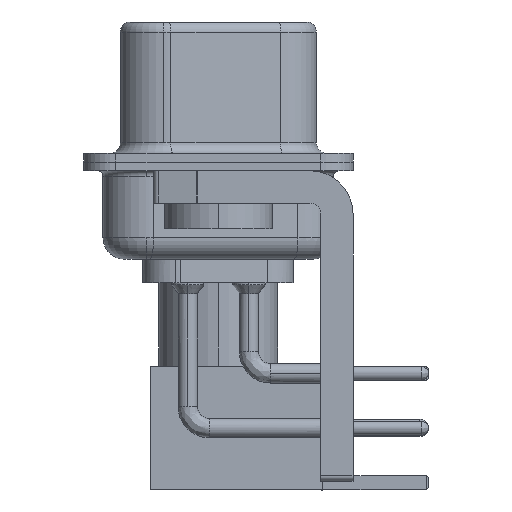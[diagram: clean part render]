
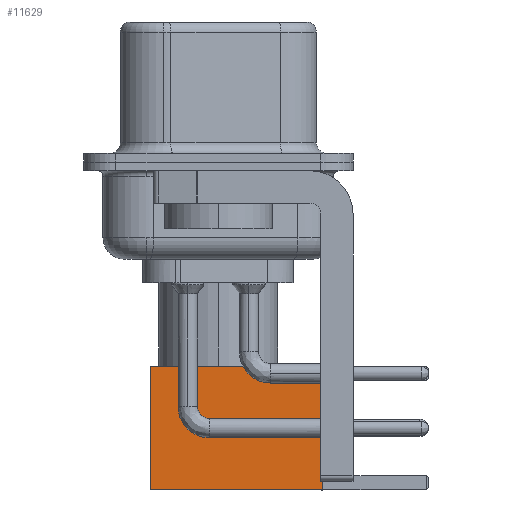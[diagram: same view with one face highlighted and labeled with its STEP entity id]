
A CAD part, left-side view. The second image highlights one B-rep face of the part: STEP entity #11629.
In plain terms, the highlighted face is planar.
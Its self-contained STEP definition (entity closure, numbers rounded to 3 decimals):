
#339 = EDGE_CURVE ( 'NONE', #1229, #10793, #1042, .T. ) ;
#400 = CARTESIAN_POINT ( 'NONE',  ( 2.875, 2.875, 0. ) ) ;
#430 = VECTOR ( 'NONE', #20013, 1000. ) ;
#1042 = LINE ( 'NONE', #17690, #430 ) ;
#1229 = VERTEX_POINT ( 'NONE', #17886 ) ;
#2007 = VECTOR ( 'NONE', #15887, 1000. ) ;
#2085 = CARTESIAN_POINT ( 'NONE',  ( 2.875, 2.875, 8. ) ) ;
#2715 = DIRECTION ( 'NONE',  ( 0., 0., 1. ) ) ;
#3270 = VERTEX_POINT ( 'NONE', #13412 ) ;
#3455 = CARTESIAN_POINT ( 'NONE',  ( 0., 2.875, 8. ) ) ;
#5475 = AXIS2_PLACEMENT_3D ( 'NONE', #400, #17496, #2715 ) ;
#10328 = LINE ( 'NONE', #3455, #12085 ) ;
#10793 = VERTEX_POINT ( 'NONE', #30194 ) ;
#11629 = ADVANCED_FACE ( 'NONE', ( #21705 ), #14875, .T. ) ;
#12078 = EDGE_CURVE ( 'NONE', #19626, #1229, #30085, .T. ) ;
#12085 = VECTOR ( 'NONE', #13126, 1000. ) ;
#12333 = LINE ( 'NONE', #14365, #27071 ) ;
#12868 = ORIENTED_EDGE ( 'NONE', *, *, #12078, .T. ) ;
#13126 = DIRECTION ( 'NONE',  ( -1., 0., 0. ) ) ;
#13412 = CARTESIAN_POINT ( 'NONE',  ( -2.875, 2.875, 8. ) ) ;
#14365 = CARTESIAN_POINT ( 'NONE',  ( -2.875, 2.875, 0. ) ) ;
#14718 = EDGE_CURVE ( 'NONE', #19626, #3270, #10328, .T. ) ;
#14875 = PLANE ( 'NONE',  #5475 ) ;
#15887 = DIRECTION ( 'NONE',  ( 0., 0., -1. ) ) ;
#16580 = ORIENTED_EDGE ( 'NONE', *, *, #339, .T. ) ;
#16824 = EDGE_CURVE ( 'NONE', #3270, #10793, #12333, .T. ) ;
#17496 = DIRECTION ( 'NONE',  ( 0., 1., 0. ) ) ;
#17690 = CARTESIAN_POINT ( 'NONE',  ( 0., 2.875, 0. ) ) ;
#17886 = CARTESIAN_POINT ( 'NONE',  ( 2.875, 2.875, 0. ) ) ;
#19626 = VERTEX_POINT ( 'NONE', #2085 ) ;
#20013 = DIRECTION ( 'NONE',  ( -1., 0., 0. ) ) ;
#20248 = CARTESIAN_POINT ( 'NONE',  ( 2.875, 2.875, 0. ) ) ;
#21345 = DIRECTION ( 'NONE',  ( 0., 0., -1. ) ) ;
#21705 = FACE_OUTER_BOUND ( 'NONE', #23923, .T. ) ;
#22665 = ORIENTED_EDGE ( 'NONE', *, *, #14718, .F. ) ;
#23923 = EDGE_LOOP ( 'NONE', ( #12868, #16580, #29776, #22665 ) ) ;
#27071 = VECTOR ( 'NONE', #21345, 1000. ) ;
#29776 = ORIENTED_EDGE ( 'NONE', *, *, #16824, .F. ) ;
#30085 = LINE ( 'NONE', #20248, #2007 ) ;
#30194 = CARTESIAN_POINT ( 'NONE',  ( -2.875, 2.875, 0. ) ) ;
